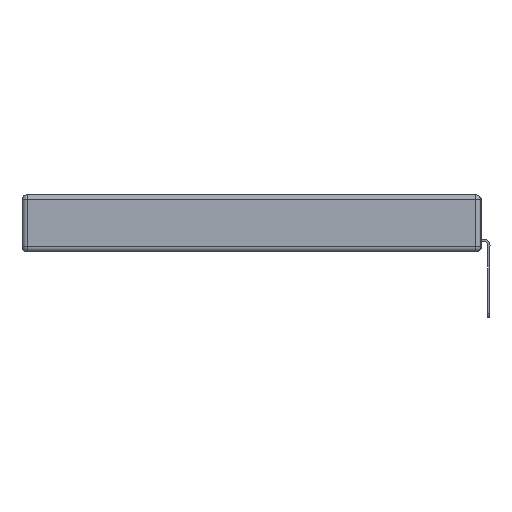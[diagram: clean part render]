
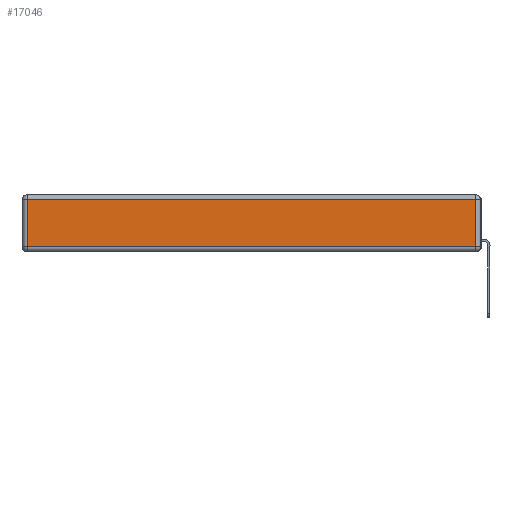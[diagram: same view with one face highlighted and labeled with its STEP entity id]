
A CAD part, left-side view. The second image highlights one B-rep face of the part: STEP entity #17046.
In plain terms, the highlighted planar face has unit normal (-1, 0, 0).
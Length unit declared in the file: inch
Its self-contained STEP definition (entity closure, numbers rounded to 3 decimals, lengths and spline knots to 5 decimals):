
#75 = DIRECTION ( 'NONE',  ( -1., 0., 0. ) ) ;
#1975 = ORIENTED_EDGE ( 'NONE', *, *, #22488, .T. ) ;
#2053 = CARTESIAN_POINT ( 'NONE',  ( 0., 0., -0.313 ) ) ;
#2282 = LINE ( 'NONE', #12481, #5066 ) ;
#2416 = DIRECTION ( 'NONE',  ( 0., 0., 1. ) ) ;
#2925 = CARTESIAN_POINT ( 'NONE',  ( 0., 2.72, -0.343 ) ) ;
#4940 = LINE ( 'NONE', #2053, #20880 ) ;
#5055 = VERTEX_POINT ( 'NONE', #26746 ) ;
#5066 = VECTOR ( 'NONE', #27986, 39.37008 ) ;
#6409 = EDGE_CURVE ( 'NONE', #15354, #24301, #20517, .T. ) ;
#8016 = CARTESIAN_POINT ( 'NONE',  ( 0., 0.03, -0.03 ) ) ;
#9196 = LINE ( 'NONE', #19103, #24098 ) ;
#9563 = DIRECTION ( 'NONE',  ( 0., 0., -1. ) ) ;
#10641 = ORIENTED_EDGE ( 'NONE', *, *, #12945, .T. ) ;
#11388 = ORIENTED_EDGE ( 'NONE', *, *, #20500, .T. ) ;
#11416 = ORIENTED_EDGE ( 'NONE', *, *, #6409, .T. ) ;
#12481 = CARTESIAN_POINT ( 'NONE',  ( 0., 2.75, -0.03 ) ) ;
#12945 = EDGE_CURVE ( 'NONE', #21750, #15354, #2282, .T. ) ;
#13346 = CARTESIAN_POINT ( 'NONE',  ( 0., 0., -0.343 ) ) ;
#14989 = VECTOR ( 'NONE', #9563, 39.37008 ) ;
#15354 = VERTEX_POINT ( 'NONE', #25219 ) ;
#15567 = PLANE ( 'NONE',  #19261 ) ;
#17046 = ADVANCED_FACE ( 'NONE', ( #22821 ), #15567, .T. ) ;
#17206 = EDGE_LOOP ( 'NONE', ( #1975, #11388, #10641, #11416 ) ) ;
#19103 = CARTESIAN_POINT ( 'NONE',  ( 0., 0.03, -0.343 ) ) ;
#19261 = AXIS2_PLACEMENT_3D ( 'NONE', #13346, #75, #2416 ) ;
#20500 = EDGE_CURVE ( 'NONE', #5055, #21750, #9196, .T. ) ;
#20517 = LINE ( 'NONE', #2925, #14989 ) ;
#20880 = VECTOR ( 'NONE', #24206, 39.37008 ) ;
#21750 = VERTEX_POINT ( 'NONE', #8016 ) ;
#22488 = EDGE_CURVE ( 'NONE', #24301, #5055, #4940, .T. ) ;
#22821 = FACE_OUTER_BOUND ( 'NONE', #17206, .T. ) ;
#23952 = DIRECTION ( 'NONE',  ( 0., 0., 1. ) ) ;
#24098 = VECTOR ( 'NONE', #23952, 39.37008 ) ;
#24206 = DIRECTION ( 'NONE',  ( 0., -1., 0. ) ) ;
#24260 = CARTESIAN_POINT ( 'NONE',  ( 0., 2.72, -0.313 ) ) ;
#24301 = VERTEX_POINT ( 'NONE', #24260 ) ;
#25219 = CARTESIAN_POINT ( 'NONE',  ( 0., 2.72, -0.03 ) ) ;
#26746 = CARTESIAN_POINT ( 'NONE',  ( 0., 0.03, -0.313 ) ) ;
#27986 = DIRECTION ( 'NONE',  ( 0., 1., 0. ) ) ;
